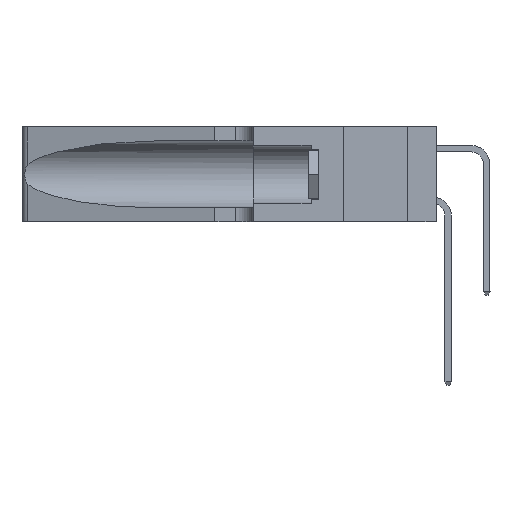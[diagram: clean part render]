
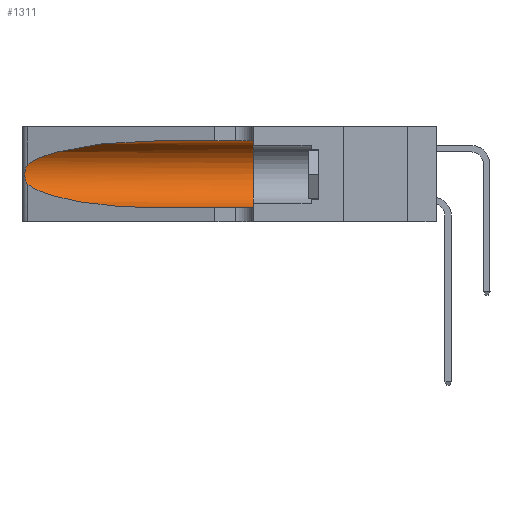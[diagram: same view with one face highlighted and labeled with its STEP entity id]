
A CAD part, left-side view. The second image highlights one B-rep face of the part: STEP entity #1311.
In plain terms, the highlighted cylindrical face has radius 3.308 mm (diameter 6.617 mm), a partial arc.
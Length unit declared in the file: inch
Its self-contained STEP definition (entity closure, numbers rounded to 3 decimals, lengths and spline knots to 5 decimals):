
#556 = CARTESIAN_POINT ( 'NONE',  ( 0.2373, 1.15595, 0.28018 ) ) ;
#986 = DIRECTION ( 'NONE',  ( 0., 0., 1. ) ) ;
#1215 = DIRECTION ( 'NONE',  ( 0., -1., 0. ) ) ;
#1311 = ADVANCED_FACE ( 'NONE', ( #38523 ), #45833, .F. ) ;
#1940 = CARTESIAN_POINT ( 'NONE',  ( 0.25487, 1.22718, 0.14631 ) ) ;
#2696 = ORIENTED_EDGE ( 'NONE', *, *, #26826, .F. ) ;
#2832 = CARTESIAN_POINT ( 'NONE',  ( 0.25487, 1.22718, 0.22369 ) ) ;
#2881 = CARTESIAN_POINT ( 'NONE',  ( 0.25487, 1.22718, 0.22369 ) ) ;
#4945 = VECTOR ( 'NONE', #43764, 39.37008 ) ;
#5002 =( BOUNDED_CURVE ( )  B_SPLINE_CURVE ( 3, ( #5268, #30542, #44799, #23566 ),
 .UNSPECIFIED., .F., .F. ) 
 B_SPLINE_CURVE_WITH_KNOTS ( ( 4, 4 ),
 ( 3.44316, 4.71239 ),
 .UNSPECIFIED. ) 
 CURVE ( )  GEOMETRIC_REPRESENTATION_ITEM ( )  RATIONAL_B_SPLINE_CURVE ( ( 1., 0.87, 0.87, 1. ) ) 
 REPRESENTATION_ITEM ( '' )  );
#5268 = CARTESIAN_POINT ( 'NONE',  ( 0.25487, 1.22718, 0.14631 ) ) ;
#6399 = CARTESIAN_POINT ( 'NONE',  ( 0.1305, 0.72297, 0.31525 ) ) ;
#6601 = CARTESIAN_POINT ( 'NONE',  ( 0.25854, 1.2359, 0.20912 ) ) ;
#6809 = EDGE_LOOP ( 'NONE', ( #45972, #15545, #34887, #19039, #2696, #17510 ) ) ;
#7832 = CARTESIAN_POINT ( 'NONE',  ( 0.18966, 0.96281, 0.31525 ) ) ;
#8445 = CARTESIAN_POINT ( 'NONE',  ( 0.1305, 0.72297, 0.05475 ) ) ;
#10287 = CARTESIAN_POINT ( 'NONE',  ( 0.26075, 1.23896, 0.19203 ) ) ;
#10714 = EDGE_CURVE ( 'NONE', #23811, #15351, #12583, .T. ) ;
#12583 = LINE ( 'NONE', #14961, #39988 ) ;
#13947 = CARTESIAN_POINT ( 'NONE',  ( 0.26017, 1.23833, 0.17102 ) ) ;
#14961 = CARTESIAN_POINT ( 'NONE',  ( 0.1305, 1.61858, 0.05475 ) ) ;
#15182 = CARTESIAN_POINT ( 'NONE',  ( 0.1305, 0.72297, 0.31525 ) ) ;
#15351 = VERTEX_POINT ( 'NONE', #30351 ) ;
#15545 = ORIENTED_EDGE ( 'NONE', *, *, #25264, .T. ) ;
#15869 = EDGE_CURVE ( 'NONE', #27010, #37419, #32570, .T. ) ;
#17009 =( BOUNDED_CURVE ( )  B_SPLINE_CURVE ( 3, ( #15182, #7832, #556, #26054 ),
 .UNSPECIFIED., .F., .F. ) 
 B_SPLINE_CURVE_WITH_KNOTS ( ( 4, 4 ),
 ( 1.5708, 2.84003 ),
 .UNSPECIFIED. ) 
 CURVE ( )  GEOMETRIC_REPRESENTATION_ITEM ( )  RATIONAL_B_SPLINE_CURVE ( ( 1., 0.87, 0.87, 1. ) ) 
 REPRESENTATION_ITEM ( '' )  );
#17510 = ORIENTED_EDGE ( 'NONE', *, *, #15869, .F. ) ;
#17618 = CARTESIAN_POINT ( 'NONE',  ( 0.25789, 1.23486, 0.15765 ) ) ;
#19039 = ORIENTED_EDGE ( 'NONE', *, *, #10714, .T. ) ;
#21262 = CARTESIAN_POINT ( 'NONE',  ( 0.25555, 1.22993, 0.14849 ) ) ;
#22537 = CARTESIAN_POINT ( 'NONE',  ( 0.1305, 1.61858, 0.31525 ) ) ;
#22874 = DIRECTION ( 'NONE',  ( 0., 1., 0. ) ) ;
#23514 = AXIS2_PLACEMENT_3D ( 'NONE', #44109, #22874, #986 ) ;
#23566 = CARTESIAN_POINT ( 'NONE',  ( 0.1305, 0.72297, 0.05475 ) ) ;
#23811 = VERTEX_POINT ( 'NONE', #8445 ) ;
#23965 = AXIS2_PLACEMENT_3D ( 'NONE', #40736, #1215, #30241 ) ;
#25264 = EDGE_CURVE ( 'NONE', #28943, #28094, #25390, .T. ) ;
#25390 = B_SPLINE_CURVE_WITH_KNOTS ( 'NONE', 3,
 ( #2881, #38730, #42345, #28248, #6601, #31799, #10287, #35318, #13947, #38885, #17618, #42502, #21262, #46120 ),
 .UNSPECIFIED., .F., .F.,
 ( 4, 2, 2, 2, 2, 2, 4 ),
 ( 0., 0.00027, 0.00053, 0.00107, 0.0016, 0.00187, 0.00214 ),
 .UNSPECIFIED. ) ;
#26054 = CARTESIAN_POINT ( 'NONE',  ( 0.25487, 1.22718, 0.22369 ) ) ;
#26083 = EDGE_CURVE ( 'NONE', #27010, #28943, #17009, .T. ) ;
#26826 = EDGE_CURVE ( 'NONE', #37419, #15351, #42689, .T. ) ;
#27010 = VERTEX_POINT ( 'NONE', #6399 ) ;
#28094 = VERTEX_POINT ( 'NONE', #1940 ) ;
#28248 = CARTESIAN_POINT ( 'NONE',  ( 0.25787, 1.23484, 0.2124 ) ) ;
#28943 = VERTEX_POINT ( 'NONE', #2832 ) ;
#30241 = DIRECTION ( 'NONE',  ( 0., 0., -1. ) ) ;
#30351 = CARTESIAN_POINT ( 'NONE',  ( 0.1305, 0.35, 0.05475 ) ) ;
#30542 = CARTESIAN_POINT ( 'NONE',  ( 0.2373, 1.15595, 0.08982 ) ) ;
#31799 = CARTESIAN_POINT ( 'NONE',  ( 0.26018, 1.23835, 0.19895 ) ) ;
#32570 = LINE ( 'NONE', #22537, #4945 ) ;
#34887 = ORIENTED_EDGE ( 'NONE', *, *, #35723, .T. ) ;
#35318 = CARTESIAN_POINT ( 'NONE',  ( 0.26075, 1.23896, 0.178 ) ) ;
#35723 = EDGE_CURVE ( 'NONE', #28094, #23811, #5002, .T. ) ;
#36316 = DIRECTION ( 'NONE',  ( 0., -1., 0. ) ) ;
#36487 = CARTESIAN_POINT ( 'NONE',  ( 0.1305, 0.35, 0.31525 ) ) ;
#37419 = VERTEX_POINT ( 'NONE', #36487 ) ;
#38523 = FACE_OUTER_BOUND ( 'NONE', #6809, .T. ) ;
#38730 = CARTESIAN_POINT ( 'NONE',  ( 0.25555, 1.22994, 0.2215 ) ) ;
#38885 = CARTESIAN_POINT ( 'NONE',  ( 0.25856, 1.23593, 0.16098 ) ) ;
#39988 = VECTOR ( 'NONE', #36316, 39.37008 ) ;
#40736 = CARTESIAN_POINT ( 'NONE',  ( 0.1305, 1.61858, 0.185 ) ) ;
#42345 = CARTESIAN_POINT ( 'NONE',  ( 0.25639, 1.23184, 0.21858 ) ) ;
#42502 = CARTESIAN_POINT ( 'NONE',  ( 0.25639, 1.23186, 0.15144 ) ) ;
#42689 = CIRCLE ( 'NONE', #23514, 0.13025 ) ;
#43764 = DIRECTION ( 'NONE',  ( 0., -1., 0. ) ) ;
#44109 = CARTESIAN_POINT ( 'NONE',  ( 0.1305, 0.35, 0.185 ) ) ;
#44799 = CARTESIAN_POINT ( 'NONE',  ( 0.18966, 0.96281, 0.05475 ) ) ;
#45833 = CYLINDRICAL_SURFACE ( 'NONE', #23965, 0.13025 ) ;
#45972 = ORIENTED_EDGE ( 'NONE', *, *, #26083, .T. ) ;
#46120 = CARTESIAN_POINT ( 'NONE',  ( 0.25487, 1.22718, 0.14631 ) ) ;
